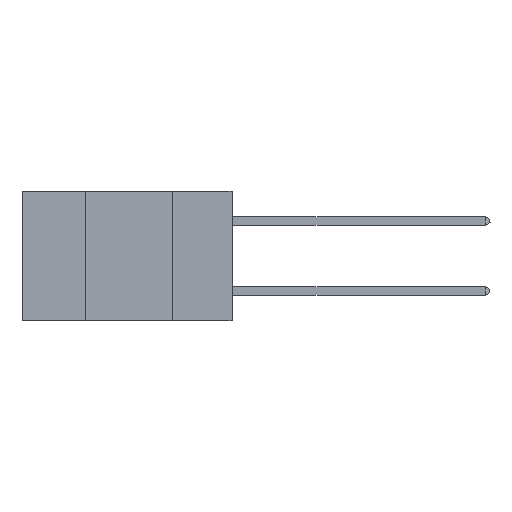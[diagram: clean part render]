
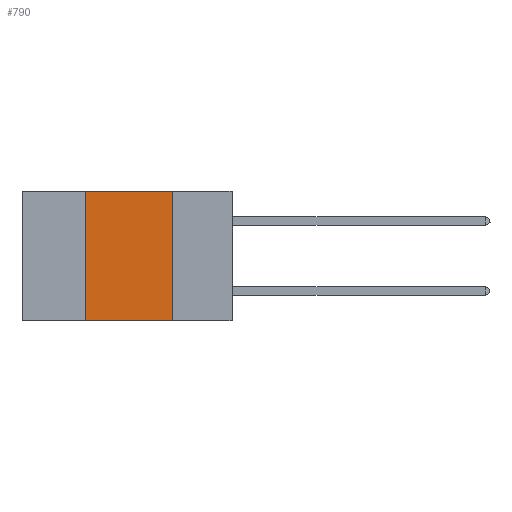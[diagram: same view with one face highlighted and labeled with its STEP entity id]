
A CAD part, left-side view. The second image highlights one B-rep face of the part: STEP entity #790.
In plain terms, the highlighted planar face has unit normal (-1, 0, 0).
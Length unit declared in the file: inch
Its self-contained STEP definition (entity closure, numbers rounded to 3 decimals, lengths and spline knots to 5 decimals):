
#766 = CARTESIAN_POINT ( 'NONE',  ( 0., 0.6, 0. ) ) ;
#790 = ADVANCED_FACE ( 'NONE', ( #5221 ), #8228, .F. ) ;
#1887 = LINE ( 'NONE', #766, #16930 ) ;
#2140 = VECTOR ( 'NONE', #14106, 39.37008 ) ;
#2317 = ORIENTED_EDGE ( 'NONE', *, *, #14007, .T. ) ;
#2335 = LINE ( 'NONE', #19544, #14754 ) ;
#3668 = VERTEX_POINT ( 'NONE', #12708 ) ;
#4718 = VERTEX_POINT ( 'NONE', #4979 ) ;
#4979 = CARTESIAN_POINT ( 'NONE',  ( 0., 0.17, 0. ) ) ;
#5221 = FACE_OUTER_BOUND ( 'NONE', #11529, .T. ) ;
#5299 = EDGE_CURVE ( 'NONE', #4718, #12016, #6291, .T. ) ;
#5648 = DIRECTION ( 'NONE',  ( 0., 0., 1. ) ) ;
#5917 = VERTEX_POINT ( 'NONE', #13025 ) ;
#5997 = CARTESIAN_POINT ( 'NONE',  ( 0., 0.6, -0.37 ) ) ;
#6291 = LINE ( 'NONE', #14253, #2140 ) ;
#6947 = DIRECTION ( 'NONE',  ( 0., 0., -1. ) ) ;
#7624 = EDGE_CURVE ( 'NONE', #3668, #5917, #2335, .T. ) ;
#7915 = CARTESIAN_POINT ( 'NONE',  ( 0., 0.17, -0.37 ) ) ;
#8228 = PLANE ( 'NONE',  #16007 ) ;
#9381 = ORIENTED_EDGE ( 'NONE', *, *, #19342, .F. ) ;
#9565 = ORIENTED_EDGE ( 'NONE', *, *, #7624, .F. ) ;
#11529 = EDGE_LOOP ( 'NONE', ( #13649, #9381, #9565, #2317 ) ) ;
#11568 = VECTOR ( 'NONE', #12213, 39.37008 ) ;
#12016 = VERTEX_POINT ( 'NONE', #7915 ) ;
#12213 = DIRECTION ( 'NONE',  ( 0., -1., 0. ) ) ;
#12708 = CARTESIAN_POINT ( 'NONE',  ( 0., 0.42, -0.37 ) ) ;
#13025 = CARTESIAN_POINT ( 'NONE',  ( 0., 0.42, 0. ) ) ;
#13649 = ORIENTED_EDGE ( 'NONE', *, *, #5299, .F. ) ;
#14007 = EDGE_CURVE ( 'NONE', #3668, #12016, #15231, .T. ) ;
#14106 = DIRECTION ( 'NONE',  ( 0., 0., -1. ) ) ;
#14253 = CARTESIAN_POINT ( 'NONE',  ( 0., 0.17, 0. ) ) ;
#14754 = VECTOR ( 'NONE', #5648, 39.37008 ) ;
#14895 = DIRECTION ( 'NONE',  ( 0., -1., 0. ) ) ;
#15231 = LINE ( 'NONE', #5997, #11568 ) ;
#16007 = AXIS2_PLACEMENT_3D ( 'NONE', #16108, #19229, #6947 ) ;
#16108 = CARTESIAN_POINT ( 'NONE',  ( 0., 0.6, 0. ) ) ;
#16930 = VECTOR ( 'NONE', #14895, 39.37008 ) ;
#19229 = DIRECTION ( 'NONE',  ( 1., 0., 0. ) ) ;
#19342 = EDGE_CURVE ( 'NONE', #5917, #4718, #1887, .T. ) ;
#19544 = CARTESIAN_POINT ( 'NONE',  ( 0., 0.42, 0. ) ) ;
